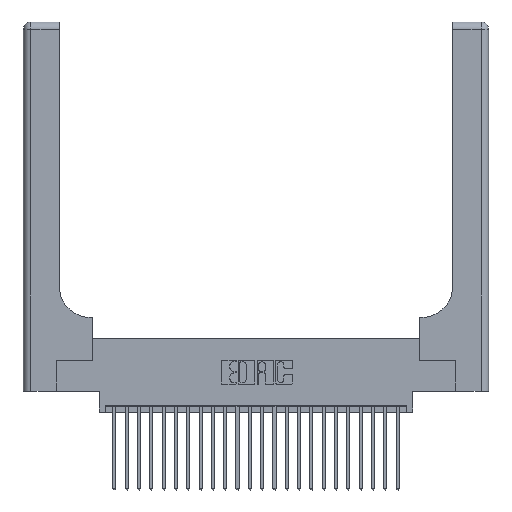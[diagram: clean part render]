
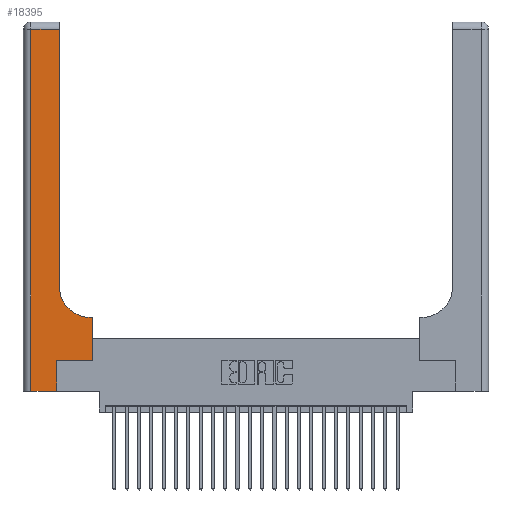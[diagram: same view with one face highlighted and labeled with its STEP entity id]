
A CAD part, top view. The second image highlights one B-rep face of the part: STEP entity #18395.
In plain terms, the highlighted planar face has unit normal (0, 0, 1).
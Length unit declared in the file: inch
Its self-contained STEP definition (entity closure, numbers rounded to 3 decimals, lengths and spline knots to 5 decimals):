
#600 = CIRCLE ( 'NONE', #15107, 0.25 ) ;
#962 = VECTOR ( 'NONE', #22899, 39.37008 ) ;
#1190 = ORIENTED_EDGE ( 'NONE', *, *, #10685, .T. ) ;
#1964 = DIRECTION ( 'NONE',  ( -1., 0., 0. ) ) ;
#3230 = CARTESIAN_POINT ( 'NONE',  ( 0.5585, 0.25, 0.37 ) ) ;
#4046 = CARTESIAN_POINT ( 'NONE',  ( 0.2915, 0.6, 0.37 ) ) ;
#5486 = VECTOR ( 'NONE', #16569, 39.37008 ) ;
#5733 = EDGE_CURVE ( 'NONE', #26185, #19761, #600, .T. ) ;
#5866 = VERTEX_POINT ( 'NONE', #3230 ) ;
#6543 = FACE_OUTER_BOUND ( 'NONE', #18584, .T. ) ;
#7023 = CARTESIAN_POINT ( 'NONE',  ( 0.5415, 0.85, 0.37 ) ) ;
#7024 = CARTESIAN_POINT ( 'NONE',  ( 0.06, 3., 0.37 ) ) ;
#8277 = CARTESIAN_POINT ( 'NONE',  ( 0.5585, 0.25, 0.37 ) ) ;
#8304 = VECTOR ( 'NONE', #9526, 39.37008 ) ;
#8597 = DIRECTION ( 'NONE',  ( 0., 0., -1. ) ) ;
#9008 = VECTOR ( 'NONE', #13228, 39.37008 ) ;
#9153 = DIRECTION ( 'NONE',  ( 1., 0., 0. ) ) ;
#9163 = CARTESIAN_POINT ( 'NONE',  ( 0.06, 2.94, 0.37 ) ) ;
#9526 = DIRECTION ( 'NONE',  ( 1., 0., 0. ) ) ;
#9645 = LINE ( 'NONE', #7024, #9008 ) ;
#9985 = EDGE_CURVE ( 'NONE', #26462, #26185, #25597, .T. ) ;
#10125 = CARTESIAN_POINT ( 'NONE',  ( 0., 0., 0.37 ) ) ;
#10164 = VECTOR ( 'NONE', #20190, 39.37008 ) ;
#10455 = VERTEX_POINT ( 'NONE', #11841 ) ;
#10685 = EDGE_CURVE ( 'NONE', #19761, #15526, #11094, .T. ) ;
#11094 = LINE ( 'NONE', #22534, #5486 ) ;
#11841 = CARTESIAN_POINT ( 'NONE',  ( 0.06, 0., 0.37 ) ) ;
#12158 = ORIENTED_EDGE ( 'NONE', *, *, #16190, .T. ) ;
#12183 = LINE ( 'NONE', #22809, #962 ) ;
#12359 = LINE ( 'NONE', #12453, #21761 ) ;
#12453 = CARTESIAN_POINT ( 'NONE',  ( 0., 2.94, 0.37 ) ) ;
#12577 = VECTOR ( 'NONE', #20441, 39.37008 ) ;
#13074 = EDGE_CURVE ( 'NONE', #21858, #10455, #9645, .T. ) ;
#13191 = LINE ( 'NONE', #15673, #8304 ) ;
#13228 = DIRECTION ( 'NONE',  ( 0., -1., 0. ) ) ;
#13989 = VERTEX_POINT ( 'NONE', #22342 ) ;
#14437 = DIRECTION ( 'NONE',  ( -1., 0., 0. ) ) ;
#14717 = CARTESIAN_POINT ( 'NONE',  ( 0., 3., 0.37 ) ) ;
#15107 = AXIS2_PLACEMENT_3D ( 'NONE', #7023, #21265, #9153 ) ;
#15252 = CARTESIAN_POINT ( 'NONE',  ( 0.5585, 0.6, 0.37 ) ) ;
#15526 = VERTEX_POINT ( 'NONE', #19558 ) ;
#15548 = VECTOR ( 'NONE', #14437, 39.37008 ) ;
#15673 = CARTESIAN_POINT ( 'NONE',  ( 0.269, 0.25, 0.37 ) ) ;
#16190 = EDGE_CURVE ( 'NONE', #13989, #5866, #13191, .T. ) ;
#16569 = DIRECTION ( 'NONE',  ( 0., 1., 0. ) ) ;
#17076 = CARTESIAN_POINT ( 'NONE',  ( 0.2915, 0.85, 0.37 ) ) ;
#17090 = ORIENTED_EDGE ( 'NONE', *, *, #13074, .T. ) ;
#17251 = CARTESIAN_POINT ( 'NONE',  ( 0.269, 0., 0.37 ) ) ;
#17275 = ORIENTED_EDGE ( 'NONE', *, *, #9985, .T. ) ;
#17581 = ORIENTED_EDGE ( 'NONE', *, *, #5733, .T. ) ;
#17884 = LINE ( 'NONE', #8277, #12577 ) ;
#18395 = ADVANCED_FACE ( 'NONE', ( #6543 ), #20750, .F. ) ;
#18584 = EDGE_LOOP ( 'NONE', ( #1190, #25371, #17090, #25832, #24890, #12158, #23074, #17275, #17581 ) ) ;
#19558 = CARTESIAN_POINT ( 'NONE',  ( 0.2915, 2.94, 0.37 ) ) ;
#19570 = EDGE_CURVE ( 'NONE', #15526, #21858, #12359, .T. ) ;
#19761 = VERTEX_POINT ( 'NONE', #17076 ) ;
#20190 = DIRECTION ( 'NONE',  ( 1., 0., 0. ) ) ;
#20421 = EDGE_CURVE ( 'NONE', #10455, #23233, #20924, .T. ) ;
#20441 = DIRECTION ( 'NONE',  ( 0., 1., 0. ) ) ;
#20750 = PLANE ( 'NONE',  #23792 ) ;
#20924 = LINE ( 'NONE', #10125, #10164 ) ;
#21265 = DIRECTION ( 'NONE',  ( 0., 0., -1. ) ) ;
#21761 = VECTOR ( 'NONE', #1964, 39.37008 ) ;
#21858 = VERTEX_POINT ( 'NONE', #9163 ) ;
#22342 = CARTESIAN_POINT ( 'NONE',  ( 0.269, 0.25, 0.37 ) ) ;
#22534 = CARTESIAN_POINT ( 'NONE',  ( 0.2915, 3., 0.37 ) ) ;
#22762 = DIRECTION ( 'NONE',  ( -1., 0., 0. ) ) ;
#22809 = CARTESIAN_POINT ( 'NONE',  ( 0.269, 0., 0.37 ) ) ;
#22899 = DIRECTION ( 'NONE',  ( 0., 1., 0. ) ) ;
#23074 = ORIENTED_EDGE ( 'NONE', *, *, #23968, .T. ) ;
#23233 = VERTEX_POINT ( 'NONE', #17251 ) ;
#23792 = AXIS2_PLACEMENT_3D ( 'NONE', #14717, #8597, #22762 ) ;
#23968 = EDGE_CURVE ( 'NONE', #5866, #26462, #17884, .T. ) ;
#24046 = CARTESIAN_POINT ( 'NONE',  ( 0.5415, 0.6, 0.37 ) ) ;
#24890 = ORIENTED_EDGE ( 'NONE', *, *, #25812, .T. ) ;
#25371 = ORIENTED_EDGE ( 'NONE', *, *, #19570, .T. ) ;
#25597 = LINE ( 'NONE', #4046, #15548 ) ;
#25812 = EDGE_CURVE ( 'NONE', #23233, #13989, #12183, .T. ) ;
#25832 = ORIENTED_EDGE ( 'NONE', *, *, #20421, .T. ) ;
#26185 = VERTEX_POINT ( 'NONE', #24046 ) ;
#26462 = VERTEX_POINT ( 'NONE', #15252 ) ;
